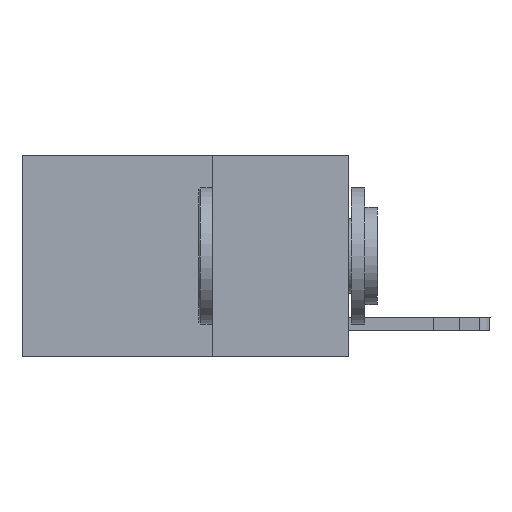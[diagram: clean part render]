
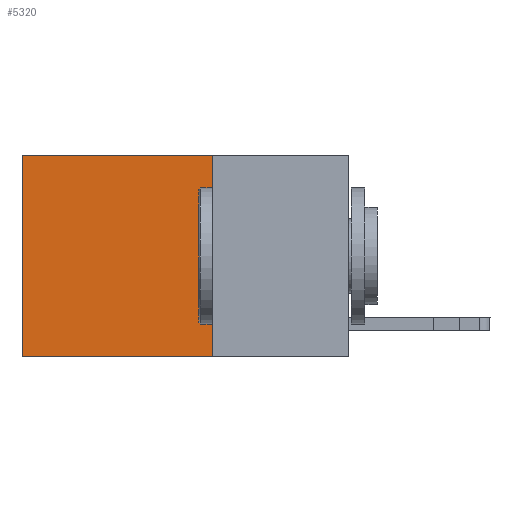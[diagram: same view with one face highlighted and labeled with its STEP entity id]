
A CAD part, left-side view. The second image highlights one B-rep face of the part: STEP entity #5320.
In plain terms, the highlighted planar face has unit normal (-1, 0, 0).
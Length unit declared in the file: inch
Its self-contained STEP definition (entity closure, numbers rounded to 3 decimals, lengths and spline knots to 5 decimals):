
#143 = DIRECTION ( 'NONE',  ( 0., 0., -1. ) ) ;
#284 = DIRECTION ( 'NONE',  ( 0., 1., 0. ) ) ;
#1306 = DIRECTION ( 'NONE',  ( 0., 0., -1. ) ) ;
#3151 = PLANE ( 'NONE',  #6773 ) ;
#3480 = LINE ( 'NONE', #12777, #3757 ) ;
#3757 = VECTOR ( 'NONE', #284, 39.37008 ) ;
#4768 = EDGE_CURVE ( 'NONE', #14974, #9028, #13120, .T. ) ;
#4803 = VECTOR ( 'NONE', #5711, 39.37008 ) ;
#5320 = ADVANCED_FACE ( 'NONE', ( #16864 ), #3151, .F. ) ;
#5444 = VERTEX_POINT ( 'NONE', #8168 ) ;
#5711 = DIRECTION ( 'NONE',  ( 0., 1., 0. ) ) ;
#6116 = LINE ( 'NONE', #15417, #15487 ) ;
#6773 = AXIS2_PLACEMENT_3D ( 'NONE', #7966, #9260, #143 ) ;
#7401 = ORIENTED_EDGE ( 'NONE', *, *, #4768, .F. ) ;
#7966 = CARTESIAN_POINT ( 'NONE',  ( 0.2625, 0.25, 0. ) ) ;
#8168 = CARTESIAN_POINT ( 'NONE',  ( 0.2625, 0.25, 0. ) ) ;
#9028 = VERTEX_POINT ( 'NONE', #12085 ) ;
#9260 = DIRECTION ( 'NONE',  ( 1., 0., 0. ) ) ;
#9268 = ORIENTED_EDGE ( 'NONE', *, *, #12351, .T. ) ;
#9574 = ORIENTED_EDGE ( 'NONE', *, *, #13294, .F. ) ;
#11040 = EDGE_LOOP ( 'NONE', ( #9268, #7401, #9574, #15033 ) ) ;
#11090 = LINE ( 'NONE', #18920, #16008 ) ;
#11588 = CARTESIAN_POINT ( 'NONE',  ( 0.2625, 0.25, -0.37 ) ) ;
#12085 = CARTESIAN_POINT ( 'NONE',  ( 0.2625, 0.6, -0.37 ) ) ;
#12351 = EDGE_CURVE ( 'NONE', #18902, #9028, #11090, .T. ) ;
#12777 = CARTESIAN_POINT ( 'NONE',  ( 0.2625, 0.25, 0. ) ) ;
#13120 = LINE ( 'NONE', #11588, #4803 ) ;
#13294 = EDGE_CURVE ( 'NONE', #5444, #14974, #6116, .T. ) ;
#13793 = CARTESIAN_POINT ( 'NONE',  ( 0.2625, 0.25, -0.37 ) ) ;
#13909 = EDGE_CURVE ( 'NONE', #5444, #18902, #3480, .T. ) ;
#14974 = VERTEX_POINT ( 'NONE', #13793 ) ;
#15033 = ORIENTED_EDGE ( 'NONE', *, *, #13909, .T. ) ;
#15417 = CARTESIAN_POINT ( 'NONE',  ( 0.2625, 0.25, 0. ) ) ;
#15487 = VECTOR ( 'NONE', #1306, 39.37008 ) ;
#16008 = VECTOR ( 'NONE', #18627, 39.37008 ) ;
#16864 = FACE_OUTER_BOUND ( 'NONE', #11040, .T. ) ;
#18627 = DIRECTION ( 'NONE',  ( 0., 0., -1. ) ) ;
#18902 = VERTEX_POINT ( 'NONE', #18993 ) ;
#18920 = CARTESIAN_POINT ( 'NONE',  ( 0.2625, 0.6, 0. ) ) ;
#18993 = CARTESIAN_POINT ( 'NONE',  ( 0.2625, 0.6, 0. ) ) ;
